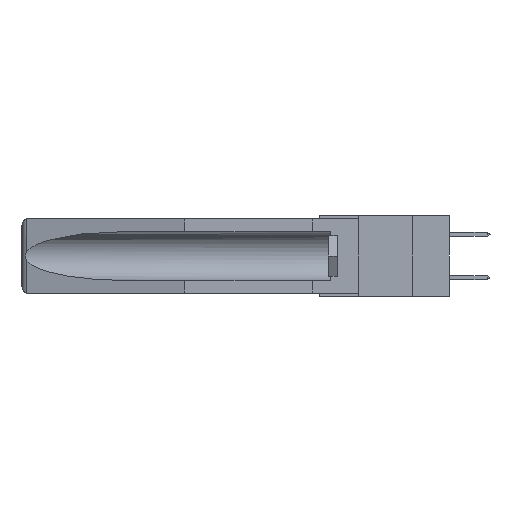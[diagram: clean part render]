
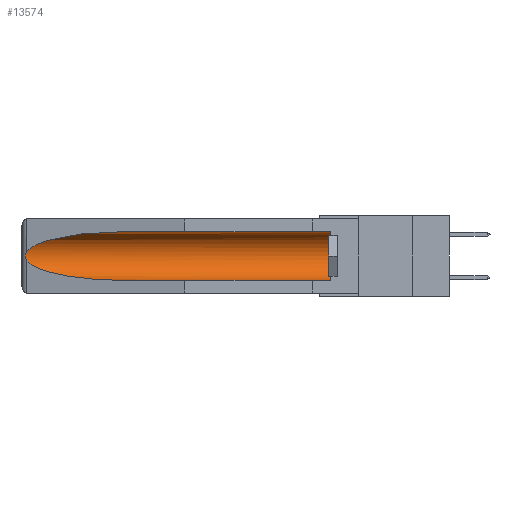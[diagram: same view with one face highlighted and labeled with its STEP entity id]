
A CAD part, left-side view. The second image highlights one B-rep face of the part: STEP entity #13574.
In plain terms, the highlighted cylindrical face has radius 2.857 mm (diameter 5.715 mm), a partial arc.
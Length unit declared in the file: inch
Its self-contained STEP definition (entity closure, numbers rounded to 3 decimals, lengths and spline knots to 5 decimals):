
#742 = DIRECTION ( 'NONE',  ( 0., 1., 0. ) ) ;
#1367 = CARTESIAN_POINT ( 'NONE',  ( 0.155, -0.30754, -0.1715 ) ) ;
#1371 = AXIS2_PLACEMENT_3D ( 'NONE', #1367, #9156, #7437 ) ;
#1447 = ORIENTED_EDGE ( 'NONE', *, *, #11456, .T. ) ;
#1882 = CARTESIAN_POINT ( 'NONE',  ( 0.26537, 1.52718, -0.19328 ) ) ;
#1924 = VERTEX_POINT ( 'NONE', #3484 ) ;
#2164 = ORIENTED_EDGE ( 'NONE', *, *, #6213, .F. ) ;
#3459 = ORIENTED_EDGE ( 'NONE', *, *, #23724, .T. ) ;
#3484 = CARTESIAN_POINT ( 'NONE',  ( 0.26537, 1.52718, -0.14972 ) ) ;
#3529 = DIRECTION ( 'NONE',  ( 0., 1., 0. ) ) ;
#3708 = VERTEX_POINT ( 'NONE', #19085 ) ;
#4110 = CARTESIAN_POINT ( 'NONE',  ( 0.25451, 1.48313, -0.24835 ) ) ;
#4183 = CARTESIAN_POINT ( 'NONE',  ( 0.26537, 1.52718, -0.19328 ) ) ;
#6157 = CARTESIAN_POINT ( 'NONE',  ( 0.26537, 1.52718, -0.19328 ) ) ;
#6213 = EDGE_CURVE ( 'NONE', #20926, #18005, #10083, .T. ) ;
#6238 = CARTESIAN_POINT ( 'NONE',  ( 0.2673, 1.53269, -0.17917 ) ) ;
#6734 = CARTESIAN_POINT ( 'NONE',  ( 0.155, 0.126, -0.1715 ) ) ;
#7197 = EDGE_CURVE ( 'NONE', #3708, #10415, #20555, .T. ) ;
#7437 = DIRECTION ( 'NONE',  ( 0., 0., 1. ) ) ;
#7442 =( BOUNDED_CURVE ( )  B_SPLINE_CURVE ( 3, ( #21686, #15982, #10482, #21438 ),
 .UNSPECIFIED., .F., .F. ) 
 B_SPLINE_CURVE_WITH_KNOTS ( ( 4, 4 ),
 ( 4.71239, 6.08839 ),
 .UNSPECIFIED. ) 
 CURVE ( )  GEOMETRIC_REPRESENTATION_ITEM ( )  RATIONAL_B_SPLINE_CURVE ( ( 1., 0.848, 0.848, 1. ) ) 
 REPRESENTATION_ITEM ( '' )  );
#7686 = CARTESIAN_POINT ( 'NONE',  ( 0.155, 0.126, -0.284 ) ) ;
#8386 = CARTESIAN_POINT ( 'NONE',  ( 0.2673, 1.5327, -0.16383 ) ) ;
#9156 = DIRECTION ( 'NONE',  ( 0., 1., 0. ) ) ;
#10083 = LINE ( 'NONE', #20312, #19138 ) ;
#10215 = CARTESIAN_POINT ( 'NONE',  ( 0.26655, 1.53094, -0.18657 ) ) ;
#10415 = VERTEX_POINT ( 'NONE', #19299 ) ;
#10482 = CARTESIAN_POINT ( 'NONE',  ( 0.25451, 1.48313, -0.09465 ) ) ;
#10517 = FACE_OUTER_BOUND ( 'NONE', #24151, .T. ) ;
#10700 = ORIENTED_EDGE ( 'NONE', *, *, #19942, .T. ) ;
#11456 = EDGE_CURVE ( 'NONE', #1924, #18551, #22754, .T. ) ;
#11493 = ORIENTED_EDGE ( 'NONE', *, *, #15887, .T. ) ;
#13388 = CARTESIAN_POINT ( 'NONE',  ( 0.21114, 1.30732, -0.284 ) ) ;
#13574 = ADVANCED_FACE ( 'NONE', ( #10517 ), #16021, .F. ) ;
#13875 = CARTESIAN_POINT ( 'NONE',  ( 0.26654, 1.53092, -0.15636 ) ) ;
#14431 = DIRECTION ( 'NONE',  ( 0., -1., 0. ) ) ;
#15082 =( BOUNDED_CURVE ( )  B_SPLINE_CURVE ( 3, ( #4183, #4110, #13388, #15322 ),
 .UNSPECIFIED., .F., .F. ) 
 B_SPLINE_CURVE_WITH_KNOTS ( ( 4, 4 ),
 ( 0.1948, 1.5708 ),
 .UNSPECIFIED. ) 
 CURVE ( )  GEOMETRIC_REPRESENTATION_ITEM ( )  RATIONAL_B_SPLINE_CURVE ( ( 1., 0.848, 0.848, 1. ) ) 
 REPRESENTATION_ITEM ( '' )  );
#15322 = CARTESIAN_POINT ( 'NONE',  ( 0.155, 1.07973, -0.284 ) ) ;
#15887 = EDGE_CURVE ( 'NONE', #10415, #1924, #7442, .T. ) ;
#15982 = CARTESIAN_POINT ( 'NONE',  ( 0.21114, 1.30732, -0.059 ) ) ;
#16021 = CYLINDRICAL_SURFACE ( 'NONE', #1371, 0.1125 ) ;
#17301 = VECTOR ( 'NONE', #742, 39.37008 ) ;
#17447 = CARTESIAN_POINT ( 'NONE',  ( 0.155, -0.30754, -0.059 ) ) ;
#18005 = VERTEX_POINT ( 'NONE', #21659 ) ;
#18551 = VERTEX_POINT ( 'NONE', #1882 ) ;
#19085 = CARTESIAN_POINT ( 'NONE',  ( 0.155, 0.126, -0.059 ) ) ;
#19138 = VECTOR ( 'NONE', #3529, 39.37008 ) ;
#19299 = CARTESIAN_POINT ( 'NONE',  ( 0.155, 1.07973, -0.059 ) ) ;
#19602 = CARTESIAN_POINT ( 'NONE',  ( 0.26537, 1.52718, -0.14972 ) ) ;
#19942 = EDGE_CURVE ( 'NONE', #20926, #3708, #23436, .T. ) ;
#20026 = DIRECTION ( 'NONE',  ( 0., 0., 1. ) ) ;
#20312 = CARTESIAN_POINT ( 'NONE',  ( 0.155, -0.30754, -0.284 ) ) ;
#20555 = LINE ( 'NONE', #17447, #17301 ) ;
#20926 = VERTEX_POINT ( 'NONE', #7686 ) ;
#21087 = AXIS2_PLACEMENT_3D ( 'NONE', #6734, #14431, #20026 ) ;
#21410 = CARTESIAN_POINT ( 'NONE',  ( 0.2675, 1.53308, -0.16763 ) ) ;
#21438 = CARTESIAN_POINT ( 'NONE',  ( 0.26537, 1.52718, -0.14972 ) ) ;
#21494 = CARTESIAN_POINT ( 'NONE',  ( 0.26597, 1.52961, -0.15275 ) ) ;
#21659 = CARTESIAN_POINT ( 'NONE',  ( 0.155, 1.07973, -0.284 ) ) ;
#21686 = CARTESIAN_POINT ( 'NONE',  ( 0.155, 1.07973, -0.059 ) ) ;
#22754 = B_SPLINE_CURVE_WITH_KNOTS ( 'NONE', 3,
 ( #19602, #21494, #13875, #8386, #21410, #23132, #6238, #10215, #23372, #6157 ),
 .UNSPECIFIED., .F., .F.,
 ( 4, 2, 2, 2, 4 ),
 ( 0., 0.00029, 0.00058, 0.00087, 0.00117 ),
 .UNSPECIFIED. ) ;
#23132 = CARTESIAN_POINT ( 'NONE',  ( 0.2675, 1.53308, -0.17534 ) ) ;
#23277 = ORIENTED_EDGE ( 'NONE', *, *, #7197, .T. ) ;
#23372 = CARTESIAN_POINT ( 'NONE',  ( 0.26597, 1.5296, -0.19026 ) ) ;
#23436 = CIRCLE ( 'NONE', #21087, 0.1125 ) ;
#23724 = EDGE_CURVE ( 'NONE', #18551, #18005, #15082, .T. ) ;
#24151 = EDGE_LOOP ( 'NONE', ( #11493, #1447, #3459, #2164, #10700, #23277 ) ) ;
